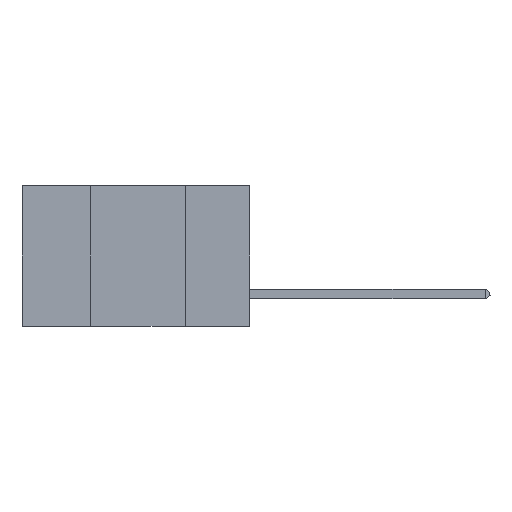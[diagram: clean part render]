
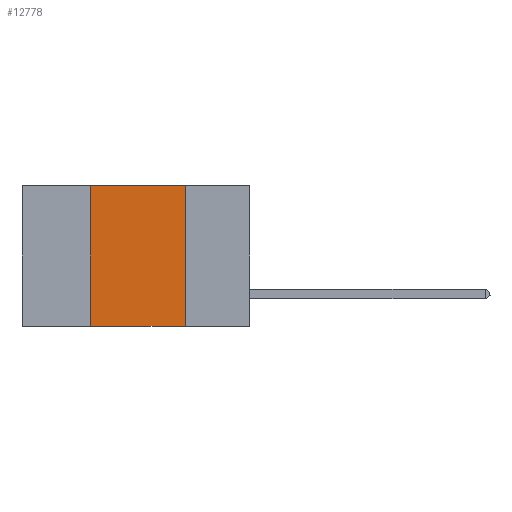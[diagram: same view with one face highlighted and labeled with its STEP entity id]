
A CAD part, left-side view. The second image highlights one B-rep face of the part: STEP entity #12778.
In plain terms, the highlighted planar face has unit normal (-1, 0, 0).
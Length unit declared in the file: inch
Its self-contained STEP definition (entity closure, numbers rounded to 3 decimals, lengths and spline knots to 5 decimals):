
#7 = ORIENTED_EDGE ( 'NONE', *, *, #7599, .T. ) ;
#160 = CARTESIAN_POINT ( 'NONE',  ( 0., 0.42, 0. ) ) ;
#171 = DIRECTION ( 'NONE',  ( 1., 0., 0. ) ) ;
#1621 = CARTESIAN_POINT ( 'NONE',  ( 0., 0.6, 0. ) ) ;
#1800 = LINE ( 'NONE', #12153, #13330 ) ;
#2288 = DIRECTION ( 'NONE',  ( 0., 0., -1. ) ) ;
#2576 = AXIS2_PLACEMENT_3D ( 'NONE', #3115, #171, #2288 ) ;
#3115 = CARTESIAN_POINT ( 'NONE',  ( 0., 0.6, 0. ) ) ;
#3190 = CARTESIAN_POINT ( 'NONE',  ( 0., 0.17, 0. ) ) ;
#3775 = CARTESIAN_POINT ( 'NONE',  ( 0., 0.6, -0.37 ) ) ;
#3912 = DIRECTION ( 'NONE',  ( 0., -1., 0. ) ) ;
#4678 = DIRECTION ( 'NONE',  ( 0., 0., 1. ) ) ;
#5583 = VERTEX_POINT ( 'NONE', #11381 ) ;
#5600 = VECTOR ( 'NONE', #4678, 39.37008 ) ;
#5687 = ORIENTED_EDGE ( 'NONE', *, *, #10319, .F. ) ;
#5818 = DIRECTION ( 'NONE',  ( 0., -1., 0. ) ) ;
#5885 = FACE_OUTER_BOUND ( 'NONE', #7045, .T. ) ;
#6070 = CARTESIAN_POINT ( 'NONE',  ( 0., 0.17, -0.37 ) ) ;
#6139 = CARTESIAN_POINT ( 'NONE',  ( 0., 0.42, -0.37 ) ) ;
#7045 = EDGE_LOOP ( 'NONE', ( #13241, #7815, #5687, #7 ) ) ;
#7198 = VECTOR ( 'NONE', #3912, 39.37008 ) ;
#7435 = PLANE ( 'NONE',  #2576 ) ;
#7501 = EDGE_CURVE ( 'NONE', #13148, #10905, #1800, .T. ) ;
#7599 = EDGE_CURVE ( 'NONE', #9623, #10905, #12448, .T. ) ;
#7815 = ORIENTED_EDGE ( 'NONE', *, *, #12726, .F. ) ;
#9623 = VERTEX_POINT ( 'NONE', #6139 ) ;
#10319 = EDGE_CURVE ( 'NONE', #9623, #5583, #12390, .T. ) ;
#10905 = VERTEX_POINT ( 'NONE', #6070 ) ;
#11381 = CARTESIAN_POINT ( 'NONE',  ( 0., 0.42, 0. ) ) ;
#11496 = VECTOR ( 'NONE', #5818, 39.37008 ) ;
#12153 = CARTESIAN_POINT ( 'NONE',  ( 0., 0.17, 0. ) ) ;
#12338 = DIRECTION ( 'NONE',  ( 0., 0., -1. ) ) ;
#12390 = LINE ( 'NONE', #160, #5600 ) ;
#12448 = LINE ( 'NONE', #3775, #7198 ) ;
#12726 = EDGE_CURVE ( 'NONE', #5583, #13148, #14431, .T. ) ;
#12778 = ADVANCED_FACE ( 'NONE', ( #5885 ), #7435, .F. ) ;
#13148 = VERTEX_POINT ( 'NONE', #3190 ) ;
#13241 = ORIENTED_EDGE ( 'NONE', *, *, #7501, .F. ) ;
#13330 = VECTOR ( 'NONE', #12338, 39.37008 ) ;
#14431 = LINE ( 'NONE', #1621, #11496 ) ;
